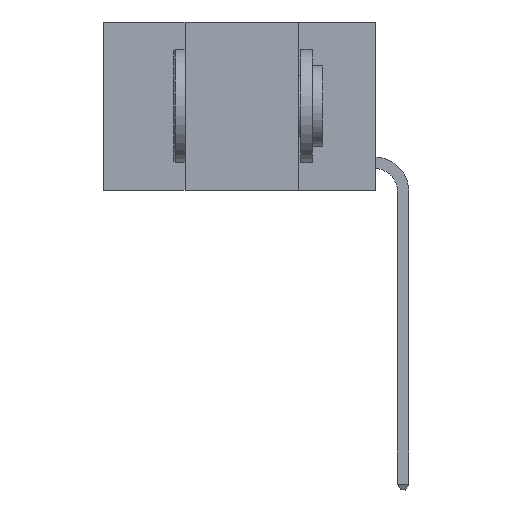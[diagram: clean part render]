
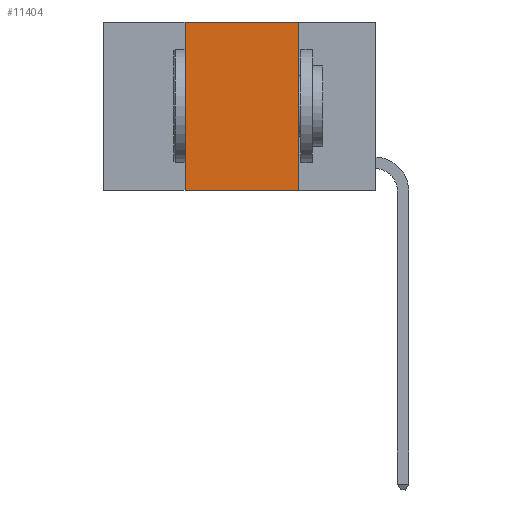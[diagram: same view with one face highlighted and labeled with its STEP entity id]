
A CAD part, left-side view. The second image highlights one B-rep face of the part: STEP entity #11404.
In plain terms, the highlighted planar face has unit normal (-1, 0, 0).
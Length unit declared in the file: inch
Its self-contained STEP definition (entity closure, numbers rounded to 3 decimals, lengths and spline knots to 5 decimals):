
#13 = VECTOR ( 'NONE', #11098, 39.37008 ) ;
#503 = LINE ( 'NONE', #13957, #13 ) ;
#521 = PLANE ( 'NONE',  #18857 ) ;
#2595 = CARTESIAN_POINT ( 'NONE',  ( 0., 0.17, 0. ) ) ;
#2624 = LINE ( 'NONE', #17273, #3114 ) ;
#3114 = VECTOR ( 'NONE', #18725, 39.37008 ) ;
#3170 = VECTOR ( 'NONE', #14008, 39.37008 ) ;
#3882 = ORIENTED_EDGE ( 'NONE', *, *, #16325, .T. ) ;
#4779 = FACE_OUTER_BOUND ( 'NONE', #7586, .T. ) ;
#5119 = EDGE_CURVE ( 'NONE', #13493, #18071, #2624, .T. ) ;
#6291 = VERTEX_POINT ( 'NONE', #17245 ) ;
#6588 = DIRECTION ( 'NONE',  ( 1., 0., 0. ) ) ;
#6967 = ORIENTED_EDGE ( 'NONE', *, *, #12773, .F. ) ;
#7176 = DIRECTION ( 'NONE',  ( 0., 0., 1. ) ) ;
#7586 = EDGE_LOOP ( 'NONE', ( #18444, #12227, #6967, #3882 ) ) ;
#10986 = CARTESIAN_POINT ( 'NONE',  ( 0., 0.6, 0. ) ) ;
#11098 = DIRECTION ( 'NONE',  ( 0., 0., -1. ) ) ;
#11404 = ADVANCED_FACE ( 'NONE', ( #4779 ), #521, .F. ) ;
#11551 = LINE ( 'NONE', #15559, #3170 ) ;
#12030 = CARTESIAN_POINT ( 'NONE',  ( 0., 0.42, 0. ) ) ;
#12052 = CARTESIAN_POINT ( 'NONE',  ( 0., 0.42, -0.37 ) ) ;
#12227 = ORIENTED_EDGE ( 'NONE', *, *, #5119, .F. ) ;
#12773 = EDGE_CURVE ( 'NONE', #12850, #13493, #17865, .T. ) ;
#12850 = VERTEX_POINT ( 'NONE', #12052 ) ;
#13493 = VERTEX_POINT ( 'NONE', #12030 ) ;
#13957 = CARTESIAN_POINT ( 'NONE',  ( 0., 0.17, 0. ) ) ;
#13968 = VECTOR ( 'NONE', #7176, 39.37008 ) ;
#14008 = DIRECTION ( 'NONE',  ( 0., -1., 0. ) ) ;
#15559 = CARTESIAN_POINT ( 'NONE',  ( 0., 0.6, -0.37 ) ) ;
#16325 = EDGE_CURVE ( 'NONE', #12850, #6291, #11551, .T. ) ;
#16869 = DIRECTION ( 'NONE',  ( 0., 0., -1. ) ) ;
#17245 = CARTESIAN_POINT ( 'NONE',  ( 0., 0.17, -0.37 ) ) ;
#17273 = CARTESIAN_POINT ( 'NONE',  ( 0., 0.6, 0. ) ) ;
#17438 = CARTESIAN_POINT ( 'NONE',  ( 0., 0.42, 0. ) ) ;
#17581 = EDGE_CURVE ( 'NONE', #18071, #6291, #503, .T. ) ;
#17865 = LINE ( 'NONE', #17438, #13968 ) ;
#18071 = VERTEX_POINT ( 'NONE', #2595 ) ;
#18444 = ORIENTED_EDGE ( 'NONE', *, *, #17581, .F. ) ;
#18725 = DIRECTION ( 'NONE',  ( 0., -1., 0. ) ) ;
#18857 = AXIS2_PLACEMENT_3D ( 'NONE', #10986, #6588, #16869 ) ;
